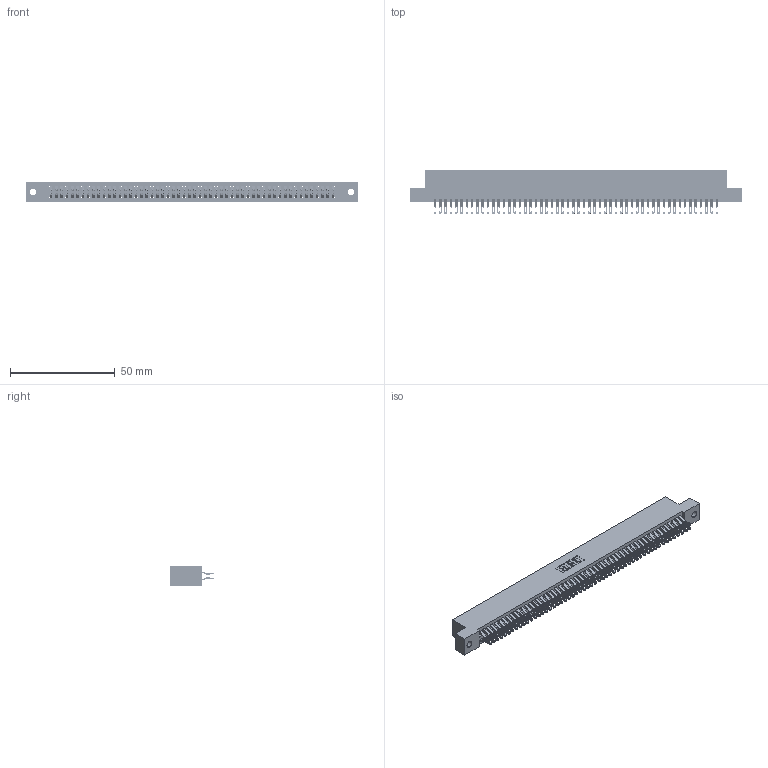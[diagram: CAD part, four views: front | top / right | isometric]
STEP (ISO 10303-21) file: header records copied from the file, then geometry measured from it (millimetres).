
FILE_DESCRIPTION (( 'STEP AP203' ), '1' );
FILE_NAME ('345-108-555-202.STEP', '2019-11-04T13:59:49', ( '' ), ( '' ), 'SwSTEP 2.0', 'SolidWorks 2016', '' );
FILE_SCHEMA (( 'CONFIG_CONTROL_DESIGN' ));
Length unit declared in the file: inch
Products named in the file (3): 345-292-001_555 Tail; 345-108-555-202; 345 Part_Flush Mounting Lugs - 0.128 Dia
Assembly tree (109 placements, depth 2):
  345-108-555-202
    345 Part_Flush Mounting Lugs - 0.128 Dia
    345-292-001_555 Tail  x108
Bounding box: 158.37 x 21.13 x 9.4 mm (x, y, z)
Volume: 15772.1 mm3; surface area: 24363 mm2
Topology: 109 solids, 109 shells, 6174 faces, 19457 edges, 12970 vertices
Faces by surface type: plane 3428, cylinder 2746
Entity records: 41083 total; most frequent: CARTESIAN_POINT 6910, ORIENTED_EDGE 6814, DIRECTION 6047, EDGE_CURVE 3407, LINE 3039, VECTOR 3039, VERTEX_POINT 2270, AXIS2_PLACEMENT_3D 1504
